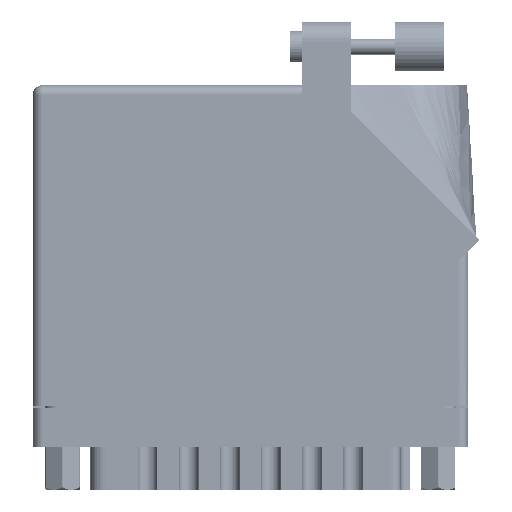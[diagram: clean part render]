
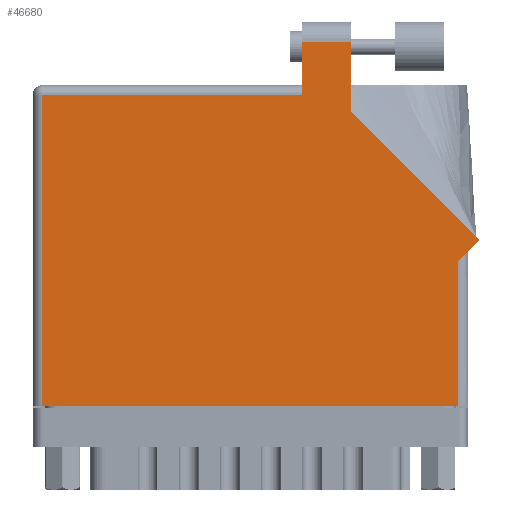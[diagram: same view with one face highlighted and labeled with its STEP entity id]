
A CAD part, front view. The second image highlights one B-rep face of the part: STEP entity #46680.
In plain terms, the highlighted face is planar.
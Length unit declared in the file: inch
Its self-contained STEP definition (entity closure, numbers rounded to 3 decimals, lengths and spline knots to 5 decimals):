
#900 = AXIS2_PLACEMENT_3D ( 'NONE', #32169, #7829, #16089 ) ;
#2870 = VERTEX_POINT ( 'NONE', #16490 ) ;
#2916 = LINE ( 'NONE', #63838, #29797 ) ;
#3032 = DIRECTION ( 'NONE',  ( -0.707, 0.707, 0. ) ) ;
#4323 = CARTESIAN_POINT ( 'NONE',  ( 2.82571, 1.05071, 0. ) ) ;
#6876 = ORIENTED_EDGE ( 'NONE', *, *, #47261, .T. ) ;
#7829 = DIRECTION ( 'NONE',  ( 0., 0., -1. ) ) ;
#7944 = VECTOR ( 'NONE', #94553, 39.37008 ) ;
#9005 = EDGE_CURVE ( 'NONE', #2870, #23973, #63449, .T. ) ;
#10325 = CARTESIAN_POINT ( 'NONE',  ( 0.062, 0., 0. ) ) ;
#11374 = CARTESIAN_POINT ( 'NONE',  ( 2.012, 1.86442, 0. ) ) ;
#12276 = CARTESIAN_POINT ( 'NONE',  ( 2.693, 0.98, 0. ) ) ;
#13094 = LINE ( 'NONE', #12276, #7944 ) ;
#13109 = VECTOR ( 'NONE', #100697, 39.37008 ) ;
#15980 = LINE ( 'NONE', #26666, #45429 ) ;
#16089 = DIRECTION ( 'NONE',  ( -1., 0., 0. ) ) ;
#16490 = CARTESIAN_POINT ( 'NONE',  ( 0.062, 0., 0. ) ) ;
#16894 = ORIENTED_EDGE ( 'NONE', *, *, #101007, .T. ) ;
#18511 = VERTEX_POINT ( 'NONE', #36302 ) ;
#19051 = CARTESIAN_POINT ( 'NONE',  ( 2.012, 1.86442, 0. ) ) ;
#21487 = CARTESIAN_POINT ( 'NONE',  ( 1.705, 1.968, 0. ) ) ;
#21519 = CARTESIAN_POINT ( 'NONE',  ( 0., 0., 0. ) ) ;
#23973 = VERTEX_POINT ( 'NONE', #67798 ) ;
#24690 = VERTEX_POINT ( 'NONE', #21487 ) ;
#26666 = CARTESIAN_POINT ( 'NONE',  ( 2.82571, 1.05071, 0. ) ) ;
#29797 = VECTOR ( 'NONE', #72060, 39.37008 ) ;
#30516 = VERTEX_POINT ( 'NONE', #92233 ) ;
#31336 = CARTESIAN_POINT ( 'NONE',  ( 1.705, 2.305, 0. ) ) ;
#32169 = CARTESIAN_POINT ( 'NONE',  ( 0., 2.03, 0. ) ) ;
#36094 = EDGE_CURVE ( 'NONE', #83444, #95717, #15980, .T. ) ;
#36302 = CARTESIAN_POINT ( 'NONE',  ( 2.693, 0.918, 0. ) ) ;
#40235 = VECTOR ( 'NONE', #75737, 39.37008 ) ;
#41677 = VECTOR ( 'NONE', #78751, 39.37008 ) ;
#45429 = VECTOR ( 'NONE', #3032, 39.37008 ) ;
#45445 = EDGE_CURVE ( 'NONE', #88578, #2870, #86339, .T. ) ;
#46680 = ADVANCED_FACE ( 'NONE', ( #86653 ), #56862, .F. ) ;
#47261 = EDGE_CURVE ( 'NONE', #59661, #30516, #59947, .T. ) ;
#47304 = LINE ( 'NONE', #103288, #61342 ) ;
#49993 = ORIENTED_EDGE ( 'NONE', *, *, #73884, .T. ) ;
#53054 = EDGE_CURVE ( 'NONE', #18511, #83444, #105018, .T. ) ;
#53274 = CARTESIAN_POINT ( 'NONE',  ( 2.755, 0.98, 0. ) ) ;
#56862 = PLANE ( 'NONE',  #900 ) ;
#59661 = VERTEX_POINT ( 'NONE', #86663 ) ;
#59947 = LINE ( 'NONE', #31336, #84281 ) ;
#60309 = ORIENTED_EDGE ( 'NONE', *, *, #62756, .T. ) ;
#61342 = VECTOR ( 'NONE', #87138, 39.37008 ) ;
#62756 = EDGE_CURVE ( 'NONE', #95717, #59661, #69346, .T. ) ;
#63449 = LINE ( 'NONE', #21519, #41677 ) ;
#63838 = CARTESIAN_POINT ( 'NONE',  ( 0., 1.968, 0. ) ) ;
#67372 = CARTESIAN_POINT ( 'NONE',  ( 0.062, 1.968, 0. ) ) ;
#67798 = CARTESIAN_POINT ( 'NONE',  ( 2.693, 0., 0. ) ) ;
#68301 = DIRECTION ( 'NONE',  ( 0.707, 0.707, 0. ) ) ;
#68382 = ORIENTED_EDGE ( 'NONE', *, *, #97785, .T. ) ;
#69346 = LINE ( 'NONE', #19051, #13109 ) ;
#72060 = DIRECTION ( 'NONE',  ( -1., 0., 0. ) ) ;
#73884 = EDGE_CURVE ( 'NONE', #23973, #18511, #13094, .T. ) ;
#75737 = DIRECTION ( 'NONE',  ( 0., -1., 0. ) ) ;
#78325 = EDGE_LOOP ( 'NONE', ( #60309, #6876, #16894, #68382, #89339, #78806, #49993, #91514, #80565 ) ) ;
#78751 = DIRECTION ( 'NONE',  ( 1., 0., 0. ) ) ;
#78806 = ORIENTED_EDGE ( 'NONE', *, *, #9005, .T. ) ;
#80565 = ORIENTED_EDGE ( 'NONE', *, *, #36094, .T. ) ;
#83444 = VERTEX_POINT ( 'NONE', #4323 ) ;
#84281 = VECTOR ( 'NONE', #104740, 39.37008 ) ;
#86339 = LINE ( 'NONE', #10325, #40235 ) ;
#86653 = FACE_OUTER_BOUND ( 'NONE', #78325, .T. ) ;
#86663 = CARTESIAN_POINT ( 'NONE',  ( 2.012, 2.305, 0. ) ) ;
#87138 = DIRECTION ( 'NONE',  ( 0., -1., 0. ) ) ;
#88578 = VERTEX_POINT ( 'NONE', #67372 ) ;
#89339 = ORIENTED_EDGE ( 'NONE', *, *, #45445, .T. ) ;
#91514 = ORIENTED_EDGE ( 'NONE', *, *, #53054, .T. ) ;
#92233 = CARTESIAN_POINT ( 'NONE',  ( 1.705, 2.305, 0. ) ) ;
#94553 = DIRECTION ( 'NONE',  ( 0., 1., 0. ) ) ;
#94724 = VECTOR ( 'NONE', #68301, 39.37008 ) ;
#95717 = VERTEX_POINT ( 'NONE', #11374 ) ;
#97785 = EDGE_CURVE ( 'NONE', #24690, #88578, #2916, .T. ) ;
#100697 = DIRECTION ( 'NONE',  ( 0., 1., 0. ) ) ;
#101007 = EDGE_CURVE ( 'NONE', #30516, #24690, #47304, .T. ) ;
#103288 = CARTESIAN_POINT ( 'NONE',  ( 1.705, 2.03, 0. ) ) ;
#104740 = DIRECTION ( 'NONE',  ( -1., 0., 0. ) ) ;
#105018 = LINE ( 'NONE', #53274, #94724 ) ;
